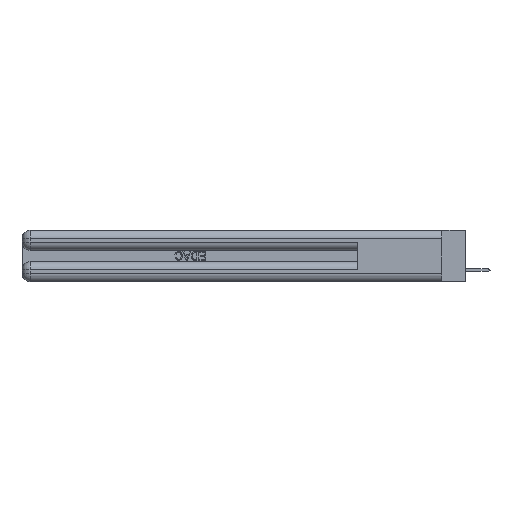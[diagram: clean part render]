
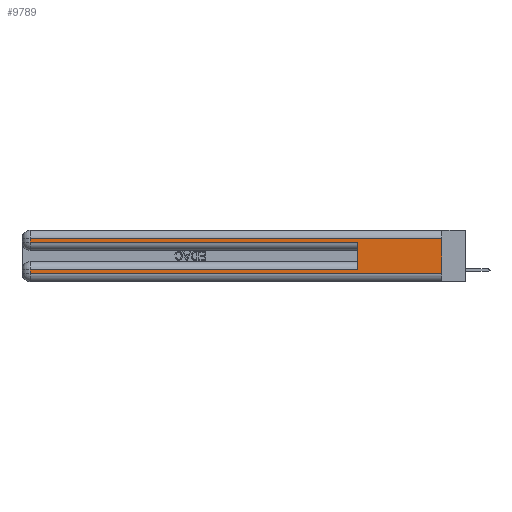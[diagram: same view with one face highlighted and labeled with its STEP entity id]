
A CAD part, left-side view. The second image highlights one B-rep face of the part: STEP entity #9789.
In plain terms, the highlighted planar face has unit normal (-1, 0, 0).
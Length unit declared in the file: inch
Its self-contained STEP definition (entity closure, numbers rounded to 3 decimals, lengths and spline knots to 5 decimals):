
#132 = LINE ( 'NONE', #22614, #32292 ) ;
#242 = VECTOR ( 'NONE', #35250, 39.37008 ) ;
#802 = ORIENTED_EDGE ( 'NONE', *, *, #8797, .T. ) ;
#1329 = ORIENTED_EDGE ( 'NONE', *, *, #25052, .T. ) ;
#1441 = DIRECTION ( 'NONE',  ( 0., 1., 0. ) ) ;
#2377 = LINE ( 'NONE', #16819, #21473 ) ;
#3603 = VERTEX_POINT ( 'NONE', #43414 ) ;
#4708 = ORIENTED_EDGE ( 'NONE', *, *, #30474, .T. ) ;
#5196 = LINE ( 'NONE', #35005, #13990 ) ;
#6772 = CARTESIAN_POINT ( 'NONE',  ( 0., 0., 0.06 ) ) ;
#7233 = CARTESIAN_POINT ( 'NONE',  ( 0., 2.94, 0.285 ) ) ;
#7355 = CARTESIAN_POINT ( 'NONE',  ( 0., 0., 0.31 ) ) ;
#7898 = PLANE ( 'NONE',  #32280 ) ;
#7980 = EDGE_CURVE ( 'NONE', #11304, #3603, #39580, .T. ) ;
#8045 = VECTOR ( 'NONE', #37065, 39.37008 ) ;
#8050 = VERTEX_POINT ( 'NONE', #40345 ) ;
#8797 = EDGE_CURVE ( 'NONE', #18476, #3603, #5196, .T. ) ;
#9692 = EDGE_CURVE ( 'NONE', #42774, #32172, #18252, .T. ) ;
#9789 = ADVANCED_FACE ( 'NONE', ( #11684 ), #7898, .F. ) ;
#10051 = VERTEX_POINT ( 'NONE', #6772 ) ;
#10915 = VECTOR ( 'NONE', #13223, 39.37008 ) ;
#11074 = CARTESIAN_POINT ( 'NONE',  ( 0., 0.6, 0.085 ) ) ;
#11247 = CARTESIAN_POINT ( 'NONE',  ( 0., 2.94, 0.06 ) ) ;
#11304 = VERTEX_POINT ( 'NONE', #11074 ) ;
#11684 = FACE_OUTER_BOUND ( 'NONE', #23668, .T. ) ;
#11710 = DIRECTION ( 'NONE',  ( 0., 0., -1. ) ) ;
#13223 = DIRECTION ( 'NONE',  ( 0., 0., -1. ) ) ;
#13619 = DIRECTION ( 'NONE',  ( 0., 0., -1. ) ) ;
#13990 = VECTOR ( 'NONE', #38032, 39.37008 ) ;
#16819 = CARTESIAN_POINT ( 'NONE',  ( 0., 0., 0.37 ) ) ;
#17153 = VECTOR ( 'NONE', #11710, 39.37008 ) ;
#18129 = DIRECTION ( 'NONE',  ( 0., 0., -1. ) ) ;
#18252 = LINE ( 'NONE', #7355, #242 ) ;
#18476 = VERTEX_POINT ( 'NONE', #7233 ) ;
#19368 = CARTESIAN_POINT ( 'NONE',  ( 0., 2.94, 0.31 ) ) ;
#19553 = DIRECTION ( 'NONE',  ( 0., -1., 0. ) ) ;
#21345 = VECTOR ( 'NONE', #19553, 39.37008 ) ;
#21473 = VECTOR ( 'NONE', #13619, 39.37008 ) ;
#22224 = ORIENTED_EDGE ( 'NONE', *, *, #35163, .T. ) ;
#22614 = CARTESIAN_POINT ( 'NONE',  ( 0., 0., 0.085 ) ) ;
#23454 = LINE ( 'NONE', #37270, #10915 ) ;
#23668 = EDGE_LOOP ( 'NONE', ( #45071, #26535, #4708, #802, #33521, #1329, #22224, #38623 ) ) ;
#25052 = EDGE_CURVE ( 'NONE', #11304, #8050, #132, .T. ) ;
#26404 = LINE ( 'NONE', #29347, #17153 ) ;
#26535 = ORIENTED_EDGE ( 'NONE', *, *, #9692, .T. ) ;
#29347 = CARTESIAN_POINT ( 'NONE',  ( 0., 2.94, 0.37 ) ) ;
#30010 = LINE ( 'NONE', #43520, #21345 ) ;
#30474 = EDGE_CURVE ( 'NONE', #32172, #18476, #26404, .T. ) ;
#31377 = EDGE_CURVE ( 'NONE', #42774, #10051, #2377, .T. ) ;
#32172 = VERTEX_POINT ( 'NONE', #19368 ) ;
#32280 = AXIS2_PLACEMENT_3D ( 'NONE', #35790, #35488, #18129 ) ;
#32292 = VECTOR ( 'NONE', #1441, 39.37008 ) ;
#33521 = ORIENTED_EDGE ( 'NONE', *, *, #7980, .F. ) ;
#34030 = VERTEX_POINT ( 'NONE', #11247 ) ;
#34556 = EDGE_CURVE ( 'NONE', #34030, #10051, #30010, .T. ) ;
#35005 = CARTESIAN_POINT ( 'NONE',  ( 0., 0., 0.285 ) ) ;
#35163 = EDGE_CURVE ( 'NONE', #8050, #34030, #23454, .T. ) ;
#35250 = DIRECTION ( 'NONE',  ( 0., 1., 0. ) ) ;
#35488 = DIRECTION ( 'NONE',  ( 1., 0., 0. ) ) ;
#35790 = CARTESIAN_POINT ( 'NONE',  ( 0., 0., 0.37 ) ) ;
#37065 = DIRECTION ( 'NONE',  ( 0., 0., 1. ) ) ;
#37270 = CARTESIAN_POINT ( 'NONE',  ( 0., 2.94, 0.37 ) ) ;
#37389 = CARTESIAN_POINT ( 'NONE',  ( 0., 0., 0.31 ) ) ;
#38032 = DIRECTION ( 'NONE',  ( 0., -1., 0. ) ) ;
#38623 = ORIENTED_EDGE ( 'NONE', *, *, #34556, .T. ) ;
#39580 = LINE ( 'NONE', #44017, #8045 ) ;
#40345 = CARTESIAN_POINT ( 'NONE',  ( 0., 2.94, 0.085 ) ) ;
#42774 = VERTEX_POINT ( 'NONE', #37389 ) ;
#43414 = CARTESIAN_POINT ( 'NONE',  ( 0., 0.6, 0.285 ) ) ;
#43520 = CARTESIAN_POINT ( 'NONE',  ( 0., 0., 0.06 ) ) ;
#44017 = CARTESIAN_POINT ( 'NONE',  ( 0., 0.6, 0.145 ) ) ;
#45071 = ORIENTED_EDGE ( 'NONE', *, *, #31377, .F. ) ;
